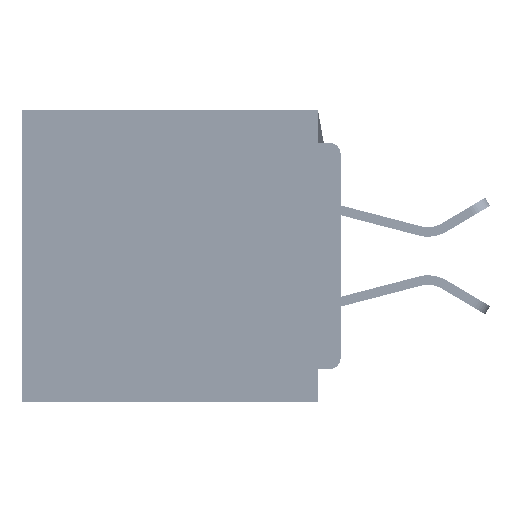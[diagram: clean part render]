
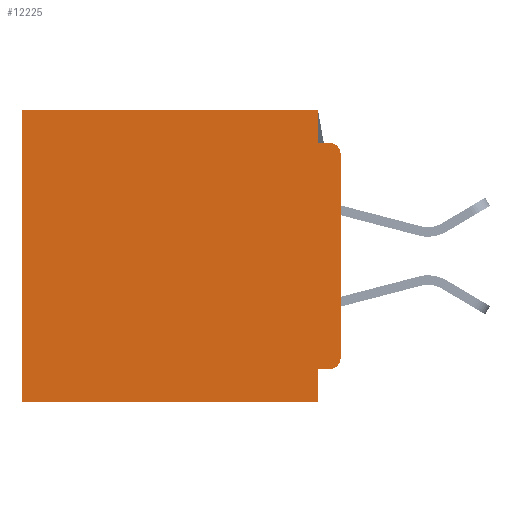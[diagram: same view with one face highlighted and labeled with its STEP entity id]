
A CAD part, left-side view. The second image highlights one B-rep face of the part: STEP entity #12225.
In plain terms, the highlighted planar face has unit normal (-1, 0, 0).
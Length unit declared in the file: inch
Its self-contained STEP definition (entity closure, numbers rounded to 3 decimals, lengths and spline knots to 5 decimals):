
#1471 = CARTESIAN_POINT ( 'NONE',  ( 0.3, 0., 0. ) ) ;
#1534 = VECTOR ( 'NONE', #31008, 39.37008 ) ;
#2807 = CARTESIAN_POINT ( 'NONE',  ( 0.3, 0., -0.355 ) ) ;
#3071 = CARTESIAN_POINT ( 'NONE',  ( 0.3, 0.015, -0.045 ) ) ;
#3942 = ORIENTED_EDGE ( 'NONE', *, *, #15286, .T. ) ;
#4787 = AXIS2_PLACEMENT_3D ( 'NONE', #24741, #62060, #30141 ) ;
#5085 = CIRCLE ( 'NONE', #6281, 0.015 ) ;
#5368 = CARTESIAN_POINT ( 'NONE',  ( 0.3, 0., -0.4 ) ) ;
#5622 = ORIENTED_EDGE ( 'NONE', *, *, #43402, .F. ) ;
#6158 = CARTESIAN_POINT ( 'NONE',  ( 0.3, 0.015, -0.06 ) ) ;
#6281 = AXIS2_PLACEMENT_3D ( 'NONE', #6158, #43616, #11511 ) ;
#7156 = VERTEX_POINT ( 'NONE', #11275 ) ;
#7295 = DIRECTION ( 'NONE',  ( 0., 1., 0. ) ) ;
#8079 = DIRECTION ( 'NONE',  ( 0., 0., -1. ) ) ;
#10320 = EDGE_CURVE ( 'NONE', #48494, #12429, #47466, .T. ) ;
#10718 = DIRECTION ( 'NONE',  ( 0., 0., -1. ) ) ;
#11275 = CARTESIAN_POINT ( 'NONE',  ( 0.3, 0.015, -0.355 ) ) ;
#11314 = CARTESIAN_POINT ( 'NONE',  ( 0.3, 0.031, -0.4 ) ) ;
#11511 = DIRECTION ( 'NONE',  ( 0., 0., -1. ) ) ;
#11878 = AXIS2_PLACEMENT_3D ( 'NONE', #5368, #42840, #10718 ) ;
#12225 = ADVANCED_FACE ( 'NONE', ( #31453 ), #26705, .F. ) ;
#12249 = ORIENTED_EDGE ( 'NONE', *, *, #32373, .F. ) ;
#12429 = VERTEX_POINT ( 'NONE', #33659 ) ;
#14771 = ORIENTED_EDGE ( 'NONE', *, *, #10320, .F. ) ;
#15286 = EDGE_CURVE ( 'NONE', #32578, #39462, #36027, .T. ) ;
#15472 = CARTESIAN_POINT ( 'NONE',  ( 0.3, 0., -0.06 ) ) ;
#17618 = EDGE_CURVE ( 'NONE', #7156, #26247, #64506, .T. ) ;
#17821 = VERTEX_POINT ( 'NONE', #68473 ) ;
#18853 = CARTESIAN_POINT ( 'NONE',  ( 0.3, 0.437, -0.4 ) ) ;
#22285 = EDGE_CURVE ( 'NONE', #42968, #32578, #29745, .T. ) ;
#24741 = CARTESIAN_POINT ( 'NONE',  ( 0.3, 0.015, -0.34 ) ) ;
#26247 = VERTEX_POINT ( 'NONE', #51580 ) ;
#26705 = PLANE ( 'NONE',  #11878 ) ;
#26722 = VECTOR ( 'NONE', #52447, 39.37008 ) ;
#28411 = CARTESIAN_POINT ( 'NONE',  ( 0.3, 0.437, -0.4 ) ) ;
#28448 = LINE ( 'NONE', #62942, #1534 ) ;
#28462 = EDGE_CURVE ( 'NONE', #48494, #32226, #5085, .T. ) ;
#29311 = EDGE_LOOP ( 'NONE', ( #14771, #46620, #12249, #64974, #30791, #3942, #5622, #51686, #60001, #55861 ) ) ;
#29745 = LINE ( 'NONE', #1471, #40587 ) ;
#30141 = DIRECTION ( 'NONE',  ( 0., 0., -1. ) ) ;
#30791 = ORIENTED_EDGE ( 'NONE', *, *, #22285, .T. ) ;
#31008 = DIRECTION ( 'NONE',  ( 0., 0., -1. ) ) ;
#31453 = FACE_OUTER_BOUND ( 'NONE', #29311, .T. ) ;
#31976 = VERTEX_POINT ( 'NONE', #11314 ) ;
#32226 = VERTEX_POINT ( 'NONE', #3071 ) ;
#32276 = EDGE_CURVE ( 'NONE', #42968, #17821, #60098, .T. ) ;
#32373 = EDGE_CURVE ( 'NONE', #17821, #32226, #67582, .T. ) ;
#32578 = VERTEX_POINT ( 'NONE', #65215 ) ;
#33659 = CARTESIAN_POINT ( 'NONE',  ( 0.3, 0., -0.34 ) ) ;
#36027 = LINE ( 'NONE', #18853, #48581 ) ;
#36131 = VECTOR ( 'NONE', #45675, 39.37008 ) ;
#39388 = CARTESIAN_POINT ( 'NONE',  ( 0.3, 0., -0.4 ) ) ;
#39462 = VERTEX_POINT ( 'NONE', #28411 ) ;
#40587 = VECTOR ( 'NONE', #54837, 39.37008 ) ;
#41961 = CARTESIAN_POINT ( 'NONE',  ( 0.3, 0., -0.045 ) ) ;
#42840 = DIRECTION ( 'NONE',  ( 1., 0., 0. ) ) ;
#42968 = VERTEX_POINT ( 'NONE', #46025 ) ;
#43402 = EDGE_CURVE ( 'NONE', #31976, #39462, #66637, .T. ) ;
#43616 = DIRECTION ( 'NONE',  ( -1., 0., 0. ) ) ;
#45675 = DIRECTION ( 'NONE',  ( 0., 1., 0. ) ) ;
#45782 = VECTOR ( 'NONE', #52616, 39.37008 ) ;
#45971 = VECTOR ( 'NONE', #46419, 39.37008 ) ;
#46025 = CARTESIAN_POINT ( 'NONE',  ( 0.3, 0.031, 0. ) ) ;
#46419 = DIRECTION ( 'NONE',  ( 0., 0., -1. ) ) ;
#46620 = ORIENTED_EDGE ( 'NONE', *, *, #28462, .T. ) ;
#47466 = LINE ( 'NONE', #57978, #45782 ) ;
#48494 = VERTEX_POINT ( 'NONE', #15472 ) ;
#48581 = VECTOR ( 'NONE', #8079, 39.37008 ) ;
#49538 = EDGE_CURVE ( 'NONE', #7156, #12429, #59807, .T. ) ;
#51580 = CARTESIAN_POINT ( 'NONE',  ( 0.3, 0.031, -0.355 ) ) ;
#51686 = ORIENTED_EDGE ( 'NONE', *, *, #55877, .F. ) ;
#52447 = DIRECTION ( 'NONE',  ( 0., -1., 0. ) ) ;
#52616 = DIRECTION ( 'NONE',  ( 0., 0., -1. ) ) ;
#54837 = DIRECTION ( 'NONE',  ( 0., 1., 0. ) ) ;
#55861 = ORIENTED_EDGE ( 'NONE', *, *, #49538, .T. ) ;
#55877 = EDGE_CURVE ( 'NONE', #26247, #31976, #28448, .T. ) ;
#56630 = CARTESIAN_POINT ( 'NONE',  ( 0.3, 0.031, 0. ) ) ;
#57978 = CARTESIAN_POINT ( 'NONE',  ( 0.3, 0., -0.4 ) ) ;
#59807 = CIRCLE ( 'NONE', #4787, 0.015 ) ;
#60001 = ORIENTED_EDGE ( 'NONE', *, *, #17618, .F. ) ;
#60098 = LINE ( 'NONE', #56630, #45971 ) ;
#62060 = DIRECTION ( 'NONE',  ( -1., 0., 0. ) ) ;
#62942 = CARTESIAN_POINT ( 'NONE',  ( 0.3, 0.031, -0.4 ) ) ;
#64506 = LINE ( 'NONE', #2807, #36131 ) ;
#64974 = ORIENTED_EDGE ( 'NONE', *, *, #32276, .F. ) ;
#64981 = VECTOR ( 'NONE', #7295, 39.37008 ) ;
#65215 = CARTESIAN_POINT ( 'NONE',  ( 0.3, 0.437, 0. ) ) ;
#66637 = LINE ( 'NONE', #39388, #64981 ) ;
#67582 = LINE ( 'NONE', #41961, #26722 ) ;
#68473 = CARTESIAN_POINT ( 'NONE',  ( 0.3, 0.031, -0.045 ) ) ;
